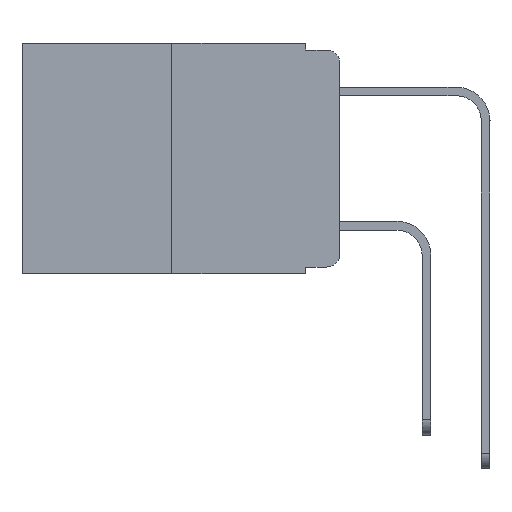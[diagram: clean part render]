
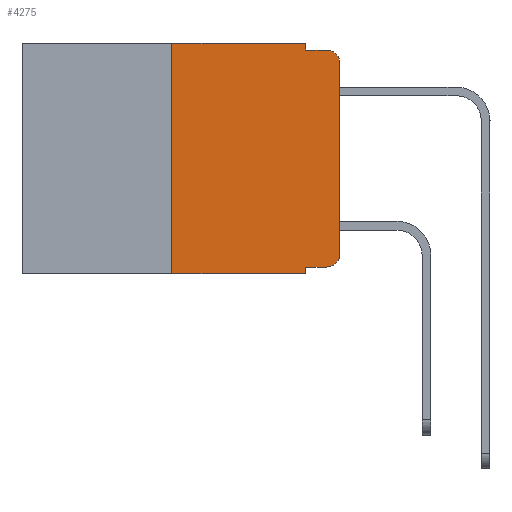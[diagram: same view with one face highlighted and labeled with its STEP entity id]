
A CAD part, left-side view. The second image highlights one B-rep face of the part: STEP entity #4275.
In plain terms, the highlighted planar face has unit normal (-1, 0, 0).
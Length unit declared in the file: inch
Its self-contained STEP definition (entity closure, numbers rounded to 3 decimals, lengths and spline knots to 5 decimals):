
#415 = LINE ( 'NONE', #25856, #20380 ) ;
#662 = CARTESIAN_POINT ( 'NONE',  ( 0., 0.051, 0. ) ) ;
#1125 = CARTESIAN_POINT ( 'NONE',  ( 0., 0.473, 0. ) ) ;
#1500 = DIRECTION ( 'NONE',  ( 0., -1., 0. ) ) ;
#2264 = DIRECTION ( 'NONE',  ( 0., 0., 1. ) ) ;
#2396 = EDGE_LOOP ( 'NONE', ( #15592, #17778, #19362, #25692, #4703, #20144, #3410, #24210, #20982, #18408 ) ) ;
#2831 = DIRECTION ( 'NONE',  ( 0., 0., -1. ) ) ;
#3041 = EDGE_CURVE ( 'NONE', #19820, #22248, #10765, .T. ) ;
#3053 = EDGE_CURVE ( 'NONE', #21171, #22061, #26445, .T. ) ;
#3213 = LINE ( 'NONE', #662, #24286 ) ;
#3410 = ORIENTED_EDGE ( 'NONE', *, *, #9215, .T. ) ;
#3877 = VERTEX_POINT ( 'NONE', #16982 ) ;
#3976 = DIRECTION ( 'NONE',  ( 0., 0., -1. ) ) ;
#4275 = ADVANCED_FACE ( 'NONE', ( #7228 ), #26327, .F. ) ;
#4703 = ORIENTED_EDGE ( 'NONE', *, *, #15948, .F. ) ;
#4791 = VERTEX_POINT ( 'NONE', #20027 ) ;
#5658 = EDGE_CURVE ( 'NONE', #12082, #4791, #22097, .T. ) ;
#6975 = LINE ( 'NONE', #25982, #22667 ) ;
#7228 = FACE_OUTER_BOUND ( 'NONE', #2396, .T. ) ;
#7347 = EDGE_CURVE ( 'NONE', #3877, #21171, #18481, .T. ) ;
#8287 = EDGE_CURVE ( 'NONE', #22648, #22061, #21067, .T. ) ;
#9215 = EDGE_CURVE ( 'NONE', #19820, #23364, #415, .T. ) ;
#9538 = CARTESIAN_POINT ( 'NONE',  ( 0., 0., -0.03 ) ) ;
#10300 = CARTESIAN_POINT ( 'NONE',  ( 0., 0.051, -0.343 ) ) ;
#10542 = CARTESIAN_POINT ( 'NONE',  ( 0., 0.051, -0.333 ) ) ;
#10765 = LINE ( 'NONE', #20618, #21068 ) ;
#11110 = CARTESIAN_POINT ( 'NONE',  ( 0., 0.02, -0.313 ) ) ;
#11216 = DIRECTION ( 'NONE',  ( -1., 0., 0. ) ) ;
#11256 = LINE ( 'NONE', #13906, #21561 ) ;
#12082 = VERTEX_POINT ( 'NONE', #12271 ) ;
#12271 = CARTESIAN_POINT ( 'NONE',  ( 0., 0.02, -0.333 ) ) ;
#12964 = VECTOR ( 'NONE', #16027, 39.37008 ) ;
#13163 = DIRECTION ( 'NONE',  ( 0., 0., -1. ) ) ;
#13906 = CARTESIAN_POINT ( 'NONE',  ( 0., 0., 0. ) ) ;
#14107 = CARTESIAN_POINT ( 'NONE',  ( 0., 0.473, 0. ) ) ;
#14482 = DIRECTION ( 'NONE',  ( 0., -1., 0. ) ) ;
#15187 = AXIS2_PLACEMENT_3D ( 'NONE', #23525, #11216, #25531 ) ;
#15592 = ORIENTED_EDGE ( 'NONE', *, *, #22745, .T. ) ;
#15948 = EDGE_CURVE ( 'NONE', #22248, #3877, #24801, .T. ) ;
#15970 = DIRECTION ( 'NONE',  ( 0., 0., 1. ) ) ;
#16027 = DIRECTION ( 'NONE',  ( 0., 0., -1. ) ) ;
#16167 = DIRECTION ( 'NONE',  ( 1., 0., 0. ) ) ;
#16982 = CARTESIAN_POINT ( 'NONE',  ( 0., 0.051, 0. ) ) ;
#17566 = DIRECTION ( 'NONE',  ( 0., -1., 0. ) ) ;
#17778 = ORIENTED_EDGE ( 'NONE', *, *, #8287, .T. ) ;
#18280 = AXIS2_PLACEMENT_3D ( 'NONE', #14107, #16167, #3976 ) ;
#18408 = ORIENTED_EDGE ( 'NONE', *, *, #5658, .T. ) ;
#18481 = LINE ( 'NONE', #22161, #12964 ) ;
#19059 = VERTEX_POINT ( 'NONE', #10542 ) ;
#19176 = EDGE_CURVE ( 'NONE', #19059, #23364, #3213, .T. ) ;
#19362 = ORIENTED_EDGE ( 'NONE', *, *, #3053, .F. ) ;
#19448 = VECTOR ( 'NONE', #17566, 39.37008 ) ;
#19820 = VERTEX_POINT ( 'NONE', #23266 ) ;
#19851 = AXIS2_PLACEMENT_3D ( 'NONE', #11110, #25405, #13163 ) ;
#19860 = DIRECTION ( 'NONE',  ( 0., -1., 0. ) ) ;
#20027 = CARTESIAN_POINT ( 'NONE',  ( 0., 0., -0.313 ) ) ;
#20144 = ORIENTED_EDGE ( 'NONE', *, *, #3041, .F. ) ;
#20242 = EDGE_CURVE ( 'NONE', #19059, #12082, #6975, .T. ) ;
#20380 = VECTOR ( 'NONE', #19860, 39.37008 ) ;
#20438 = VECTOR ( 'NONE', #14482, 39.37008 ) ;
#20618 = CARTESIAN_POINT ( 'NONE',  ( 0., 0.25, 0. ) ) ;
#20701 = CARTESIAN_POINT ( 'NONE',  ( 0., 0.051, -0.01 ) ) ;
#20982 = ORIENTED_EDGE ( 'NONE', *, *, #20242, .T. ) ;
#21067 = CIRCLE ( 'NONE', #15187, 0.02 ) ;
#21068 = VECTOR ( 'NONE', #2264, 39.37008 ) ;
#21171 = VERTEX_POINT ( 'NONE', #22967 ) ;
#21561 = VECTOR ( 'NONE', #15970, 39.37008 ) ;
#22061 = VERTEX_POINT ( 'NONE', #25988 ) ;
#22097 = CIRCLE ( 'NONE', #19851, 0.02 ) ;
#22161 = CARTESIAN_POINT ( 'NONE',  ( 0., 0.051, 0. ) ) ;
#22248 = VERTEX_POINT ( 'NONE', #24657 ) ;
#22648 = VERTEX_POINT ( 'NONE', #9538 ) ;
#22667 = VECTOR ( 'NONE', #1500, 39.37008 ) ;
#22745 = EDGE_CURVE ( 'NONE', #4791, #22648, #11256, .T. ) ;
#22967 = CARTESIAN_POINT ( 'NONE',  ( 0., 0.051, -0.01 ) ) ;
#23266 = CARTESIAN_POINT ( 'NONE',  ( 0., 0.25, -0.343 ) ) ;
#23364 = VERTEX_POINT ( 'NONE', #10300 ) ;
#23525 = CARTESIAN_POINT ( 'NONE',  ( 0., 0.02, -0.03 ) ) ;
#24210 = ORIENTED_EDGE ( 'NONE', *, *, #19176, .F. ) ;
#24286 = VECTOR ( 'NONE', #2831, 39.37008 ) ;
#24657 = CARTESIAN_POINT ( 'NONE',  ( 0., 0.25, 0. ) ) ;
#24801 = LINE ( 'NONE', #1125, #19448 ) ;
#25405 = DIRECTION ( 'NONE',  ( -1., 0., 0. ) ) ;
#25531 = DIRECTION ( 'NONE',  ( 0., 0., -1. ) ) ;
#25692 = ORIENTED_EDGE ( 'NONE', *, *, #7347, .F. ) ;
#25856 = CARTESIAN_POINT ( 'NONE',  ( 0., 0.473, -0.343 ) ) ;
#25982 = CARTESIAN_POINT ( 'NONE',  ( 0., 0.051, -0.333 ) ) ;
#25988 = CARTESIAN_POINT ( 'NONE',  ( 0., 0.02, -0.01 ) ) ;
#26327 = PLANE ( 'NONE',  #18280 ) ;
#26445 = LINE ( 'NONE', #20701, #20438 ) ;
